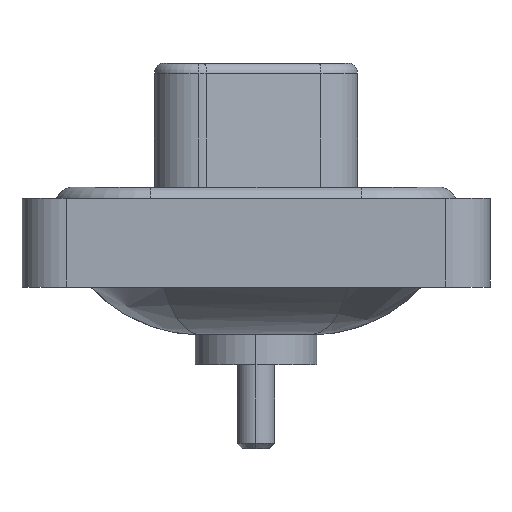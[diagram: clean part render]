
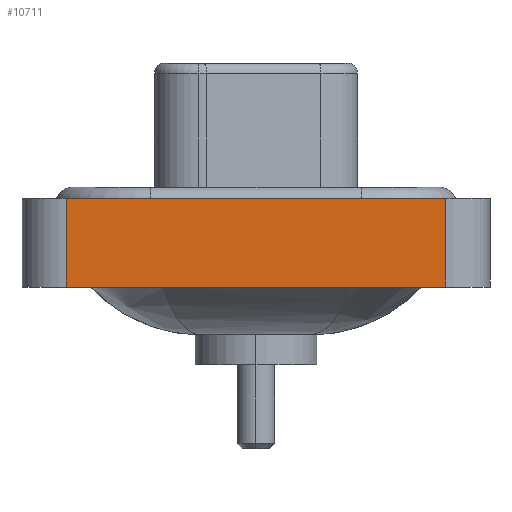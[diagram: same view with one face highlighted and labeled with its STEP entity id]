
A CAD part, left-side view. The second image highlights one B-rep face of the part: STEP entity #10711.
In plain terms, the highlighted planar face has unit normal (-1, 0, 0).
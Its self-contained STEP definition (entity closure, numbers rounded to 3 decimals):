
#607 = CARTESIAN_POINT ( 'NONE',  ( -7.3, 8.55, 0.4 ) ) ;
#1309 = ORIENTED_EDGE ( 'NONE', *, *, #13834, .T. ) ;
#1593 = VERTEX_POINT ( 'NONE', #4472 ) ;
#1619 = VERTEX_POINT ( 'NONE', #8332 ) ;
#2109 = LINE ( 'NONE', #7190, #7926 ) ;
#2239 = DIRECTION ( 'NONE',  ( 0., 0., 1. ) ) ;
#2581 = LINE ( 'NONE', #3834, #6580 ) ;
#3238 = DIRECTION ( 'NONE',  ( 0., -1., 0. ) ) ;
#3285 = PLANE ( 'NONE',  #11150 ) ;
#3611 = ORIENTED_EDGE ( 'NONE', *, *, #6056, .F. ) ;
#3834 = CARTESIAN_POINT ( 'NONE',  ( -7.3, -8.55, -3.6 ) ) ;
#4452 = VERTEX_POINT ( 'NONE', #607 ) ;
#4472 = CARTESIAN_POINT ( 'NONE',  ( -7.3, 8.55, -3.6 ) ) ;
#4564 = CARTESIAN_POINT ( 'NONE',  ( -7.3, 8.55, -3.6 ) ) ;
#5835 = LINE ( 'NONE', #4564, #12236 ) ;
#5869 = CARTESIAN_POINT ( 'NONE',  ( -7.3, -8.55, -3.6 ) ) ;
#5958 = DIRECTION ( 'NONE',  ( 0., -1., 0. ) ) ;
#6056 = EDGE_CURVE ( 'NONE', #4452, #1619, #14598, .T. ) ;
#6475 = VERTEX_POINT ( 'NONE', #12668 ) ;
#6580 = VECTOR ( 'NONE', #10395, 1000. ) ;
#7190 = CARTESIAN_POINT ( 'NONE',  ( -7.3, -8.55, -3.6 ) ) ;
#7926 = VECTOR ( 'NONE', #5958, 1000. ) ;
#8025 = ORIENTED_EDGE ( 'NONE', *, *, #12833, .T. ) ;
#8332 = CARTESIAN_POINT ( 'NONE',  ( -7.3, -8.55, 0.4 ) ) ;
#9024 = ORIENTED_EDGE ( 'NONE', *, *, #16395, .F. ) ;
#9385 = VECTOR ( 'NONE', #3238, 1000. ) ;
#9458 = FACE_OUTER_BOUND ( 'NONE', #13641, .T. ) ;
#10395 = DIRECTION ( 'NONE',  ( 0., 0., 1. ) ) ;
#10711 = ADVANCED_FACE ( 'NONE', ( #9458 ), #3285, .T. ) ;
#10935 = DIRECTION ( 'NONE',  ( 0., 0., 1. ) ) ;
#11150 = AXIS2_PLACEMENT_3D ( 'NONE', #5869, #13575, #10935 ) ;
#12236 = VECTOR ( 'NONE', #2239, 1000. ) ;
#12668 = CARTESIAN_POINT ( 'NONE',  ( -7.3, -8.55, -3.6 ) ) ;
#12833 = EDGE_CURVE ( 'NONE', #1593, #6475, #2109, .T. ) ;
#13575 = DIRECTION ( 'NONE',  ( -1., 0., 0. ) ) ;
#13641 = EDGE_LOOP ( 'NONE', ( #1309, #3611, #9024, #8025 ) ) ;
#13834 = EDGE_CURVE ( 'NONE', #6475, #1619, #2581, .T. ) ;
#14598 = LINE ( 'NONE', #15610, #9385 ) ;
#15610 = CARTESIAN_POINT ( 'NONE',  ( -7.3, -8.55, 0.4 ) ) ;
#16395 = EDGE_CURVE ( 'NONE', #1593, #4452, #5835, .T. ) ;
